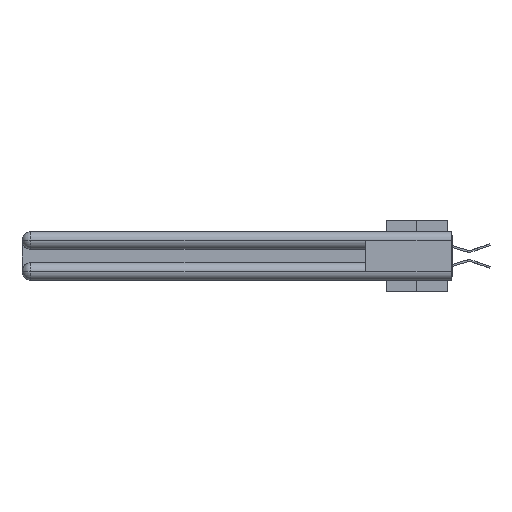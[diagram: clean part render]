
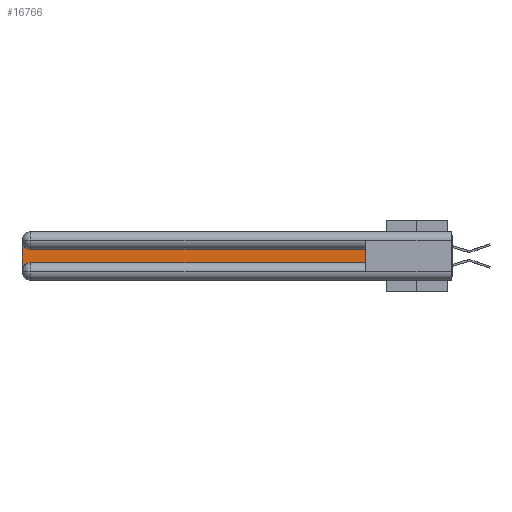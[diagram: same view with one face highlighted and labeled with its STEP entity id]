
A CAD part, left-side view. The second image highlights one B-rep face of the part: STEP entity #16766.
In plain terms, the highlighted planar face has unit normal (-1, 0, 0).
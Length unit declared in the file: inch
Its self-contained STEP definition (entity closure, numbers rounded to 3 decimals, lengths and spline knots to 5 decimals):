
#257 = ORIENTED_EDGE ( 'NONE', *, *, #16821, .T. ) ;
#2339 = EDGE_CURVE ( 'NONE', #26620, #27201, #6715, .T. ) ;
#2643 = FACE_OUTER_BOUND ( 'NONE', #33871, .T. ) ;
#2981 = VERTEX_POINT ( 'NONE', #10554 ) ;
#4207 = CARTESIAN_POINT ( 'NONE',  ( 0.075, 2.94, -0.0625 ) ) ;
#4226 = EDGE_CURVE ( 'NONE', #18794, #33468, #33080, .T. ) ;
#6564 = DIRECTION ( 'NONE',  ( 1., 0., 0. ) ) ;
#6715 = CIRCLE ( 'NONE', #25220, 0.06 ) ;
#7415 = DIRECTION ( 'NONE',  ( 0., -1., 0. ) ) ;
#7503 = VECTOR ( 'NONE', #35280, 39.37008 ) ;
#9611 = EDGE_CURVE ( 'NONE', #33468, #27499, #16839, .T. ) ;
#10386 = DIRECTION ( 'NONE',  ( 1., 0., 0. ) ) ;
#10554 = CARTESIAN_POINT ( 'NONE',  ( 0.075, 3., -0.0625 ) ) ;
#11988 = VECTOR ( 'NONE', #12734, 39.37008 ) ;
#12611 = CARTESIAN_POINT ( 'NONE',  ( 0.075, 0.6, -0.1225 ) ) ;
#12734 = DIRECTION ( 'NONE',  ( 0., 1., 0. ) ) ;
#13929 = CARTESIAN_POINT ( 'NONE',  ( 0.075, 0.6, -0.2175 ) ) ;
#14214 = VECTOR ( 'NONE', #7415, 39.37008 ) ;
#14767 = CARTESIAN_POINT ( 'NONE',  ( 0.075, 0.6, -0.1225 ) ) ;
#15436 = DIRECTION ( 'NONE',  ( 0., 0., -1. ) ) ;
#16104 = ORIENTED_EDGE ( 'NONE', *, *, #21817, .T. ) ;
#16766 = ADVANCED_FACE ( 'NONE', ( #2643 ), #29034, .F. ) ;
#16821 = EDGE_CURVE ( 'NONE', #27201, #18794, #20498, .T. ) ;
#16839 = LINE ( 'NONE', #14767, #11988 ) ;
#17048 = EDGE_CURVE ( 'NONE', #2981, #26620, #29185, .T. ) ;
#17335 = CARTESIAN_POINT ( 'NONE',  ( 0.075, 0.6, -0.2175 ) ) ;
#18065 = VECTOR ( 'NONE', #15436, 39.37008 ) ;
#18224 = ORIENTED_EDGE ( 'NONE', *, *, #17048, .T. ) ;
#18794 = VERTEX_POINT ( 'NONE', #17335 ) ;
#19729 = DIRECTION ( 'NONE',  ( 0., 0., -1. ) ) ;
#20498 = LINE ( 'NONE', #25909, #14214 ) ;
#21817 = EDGE_CURVE ( 'NONE', #27499, #2981, #28010, .T. ) ;
#24053 = ORIENTED_EDGE ( 'NONE', *, *, #4226, .T. ) ;
#24591 = CARTESIAN_POINT ( 'NONE',  ( 0.075, 3., -0.2175 ) ) ;
#25049 = CARTESIAN_POINT ( 'NONE',  ( 0.075, 2.94, -0.2775 ) ) ;
#25149 = AXIS2_PLACEMENT_3D ( 'NONE', #37564, #38385, #28182 ) ;
#25220 = AXIS2_PLACEMENT_3D ( 'NONE', #25049, #6564, #35065 ) ;
#25909 = CARTESIAN_POINT ( 'NONE',  ( 0.075, 0.6, -0.2175 ) ) ;
#26620 = VERTEX_POINT ( 'NONE', #33907 ) ;
#27201 = VERTEX_POINT ( 'NONE', #32805 ) ;
#27499 = VERTEX_POINT ( 'NONE', #38134 ) ;
#28010 = CIRCLE ( 'NONE', #39610, 0.06 ) ;
#28182 = DIRECTION ( 'NONE',  ( 0., 0., -1. ) ) ;
#29034 = PLANE ( 'NONE',  #25149 ) ;
#29185 = LINE ( 'NONE', #24591, #18065 ) ;
#32135 = ORIENTED_EDGE ( 'NONE', *, *, #9611, .T. ) ;
#32805 = CARTESIAN_POINT ( 'NONE',  ( 0.075, 2.94, -0.2175 ) ) ;
#33080 = LINE ( 'NONE', #13929, #7503 ) ;
#33468 = VERTEX_POINT ( 'NONE', #12611 ) ;
#33871 = EDGE_LOOP ( 'NONE', ( #32135, #16104, #18224, #35037, #257, #24053 ) ) ;
#33907 = CARTESIAN_POINT ( 'NONE',  ( 0.075, 3., -0.2775 ) ) ;
#35037 = ORIENTED_EDGE ( 'NONE', *, *, #2339, .T. ) ;
#35065 = DIRECTION ( 'NONE',  ( 0., 0., -1. ) ) ;
#35280 = DIRECTION ( 'NONE',  ( 0., 0., 1. ) ) ;
#37564 = CARTESIAN_POINT ( 'NONE',  ( 0.075, 3., -0.1225 ) ) ;
#38134 = CARTESIAN_POINT ( 'NONE',  ( 0.075, 2.94, -0.1225 ) ) ;
#38385 = DIRECTION ( 'NONE',  ( 1., 0., 0. ) ) ;
#39610 = AXIS2_PLACEMENT_3D ( 'NONE', #4207, #10386, #19729 ) ;
